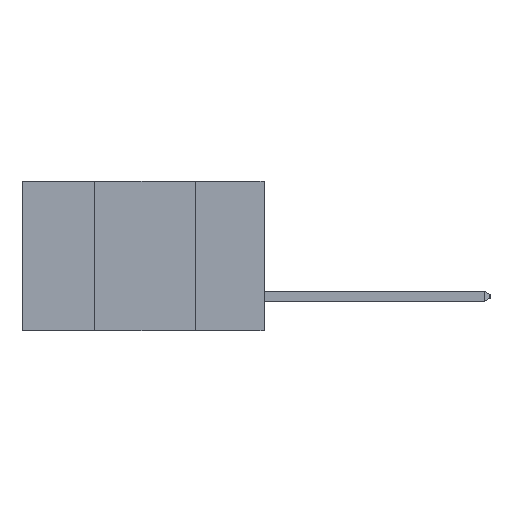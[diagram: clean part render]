
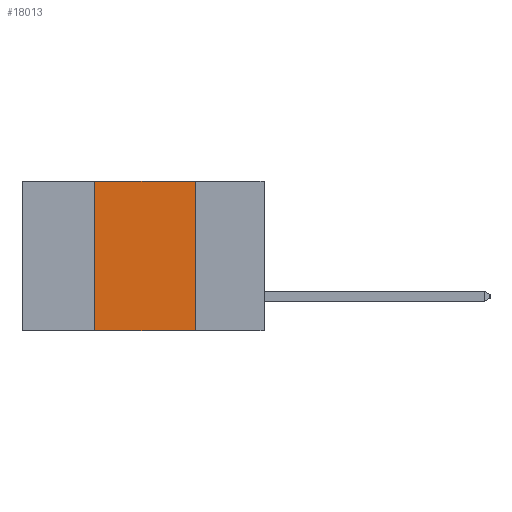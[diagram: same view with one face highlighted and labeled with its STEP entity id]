
A CAD part, left-side view. The second image highlights one B-rep face of the part: STEP entity #18013.
In plain terms, the highlighted planar face has unit normal (-1, 0, 0).
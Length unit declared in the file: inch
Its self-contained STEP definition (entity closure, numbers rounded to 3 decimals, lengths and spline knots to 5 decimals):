
#2278 = LINE ( 'NONE', #17141, #13731 ) ;
#2292 = CARTESIAN_POINT ( 'NONE',  ( 0., 0.17, -0.37 ) ) ;
#2724 = LINE ( 'NONE', #22571, #14199 ) ;
#2826 = ORIENTED_EDGE ( 'NONE', *, *, #26797, .F. ) ;
#3472 = LINE ( 'NONE', #12784, #14933 ) ;
#3798 = VERTEX_POINT ( 'NONE', #4688 ) ;
#4688 = CARTESIAN_POINT ( 'NONE',  ( 0., 0.42, -0.37 ) ) ;
#9487 = VERTEX_POINT ( 'NONE', #20707 ) ;
#10784 = CARTESIAN_POINT ( 'NONE',  ( 0., 0.6, 0. ) ) ;
#12697 = VERTEX_POINT ( 'NONE', #2292 ) ;
#12784 = CARTESIAN_POINT ( 'NONE',  ( 0., 0.6, -0.37 ) ) ;
#12963 = EDGE_CURVE ( 'NONE', #9487, #26561, #25228, .T. ) ;
#13105 = DIRECTION ( 'NONE',  ( 1., 0., 0. ) ) ;
#13731 = VECTOR ( 'NONE', #19335, 39.37008 ) ;
#14199 = VECTOR ( 'NONE', #24777, 39.37008 ) ;
#14933 = VECTOR ( 'NONE', #15046, 39.37008 ) ;
#15046 = DIRECTION ( 'NONE',  ( 0., -1., 0. ) ) ;
#15437 = ORIENTED_EDGE ( 'NONE', *, *, #12963, .F. ) ;
#16767 = ORIENTED_EDGE ( 'NONE', *, *, #28179, .F. ) ;
#16783 = DIRECTION ( 'NONE',  ( 0., -1., 0. ) ) ;
#17141 = CARTESIAN_POINT ( 'NONE',  ( 0., 0.17, 0. ) ) ;
#18013 = ADVANCED_FACE ( 'NONE', ( #20881 ), #24090, .F. ) ;
#19335 = DIRECTION ( 'NONE',  ( 0., 0., -1. ) ) ;
#20707 = CARTESIAN_POINT ( 'NONE',  ( 0., 0.42, 0. ) ) ;
#20881 = FACE_OUTER_BOUND ( 'NONE', #25180, .T. ) ;
#21593 = CARTESIAN_POINT ( 'NONE',  ( 0., 0.17, 0. ) ) ;
#22292 = ORIENTED_EDGE ( 'NONE', *, *, #25341, .T. ) ;
#22571 = CARTESIAN_POINT ( 'NONE',  ( 0., 0.42, 0. ) ) ;
#23303 = CARTESIAN_POINT ( 'NONE',  ( 0., 0.6, 0. ) ) ;
#24090 = PLANE ( 'NONE',  #28891 ) ;
#24534 = VECTOR ( 'NONE', #16783, 39.37008 ) ;
#24777 = DIRECTION ( 'NONE',  ( 0., 0., 1. ) ) ;
#25180 = EDGE_LOOP ( 'NONE', ( #16767, #15437, #2826, #22292 ) ) ;
#25228 = LINE ( 'NONE', #23303, #24534 ) ;
#25341 = EDGE_CURVE ( 'NONE', #3798, #12697, #3472, .T. ) ;
#26561 = VERTEX_POINT ( 'NONE', #21593 ) ;
#26797 = EDGE_CURVE ( 'NONE', #3798, #9487, #2724, .T. ) ;
#28179 = EDGE_CURVE ( 'NONE', #26561, #12697, #2278, .T. ) ;
#28389 = DIRECTION ( 'NONE',  ( 0., 0., -1. ) ) ;
#28891 = AXIS2_PLACEMENT_3D ( 'NONE', #10784, #13105, #28389 ) ;
